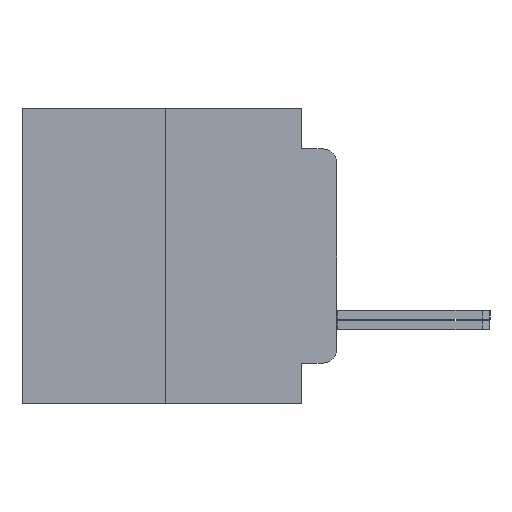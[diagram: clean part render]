
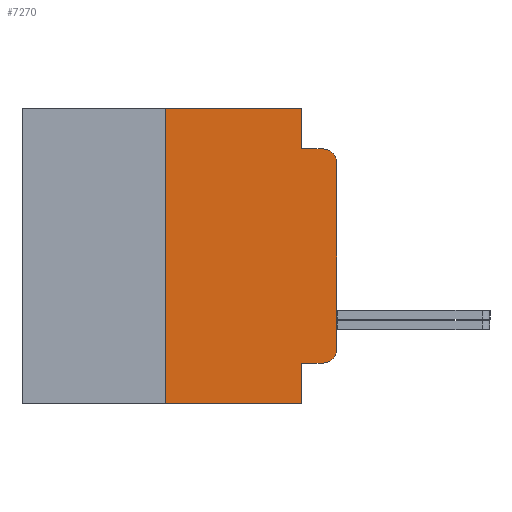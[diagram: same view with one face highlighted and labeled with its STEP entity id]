
A CAD part, left-side view. The second image highlights one B-rep face of the part: STEP entity #7270.
In plain terms, the highlighted planar face has unit normal (-1, 0, 0).
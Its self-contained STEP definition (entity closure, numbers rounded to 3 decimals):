
#16 = ORIENTED_EDGE ( 'NONE', *, *, #16278, .F. ) ;
#500 = VECTOR ( 'NONE', #19968, 1000. ) ;
#1050 = VERTEX_POINT ( 'NONE', #5140 ) ;
#1123 = DIRECTION ( 'NONE',  ( -1., 0., 0. ) ) ;
#1240 = LINE ( 'NONE', #16425, #26227 ) ;
#1304 = CARTESIAN_POINT ( 'NONE',  ( -75.603, 0.508, 3.975 ) ) ;
#1332 = DIRECTION ( 'NONE',  ( 0., 0., -1. ) ) ;
#1714 = VECTOR ( 'NONE', #20306, 1000. ) ;
#1726 = EDGE_LOOP ( 'NONE', ( #14615, #13781, #3419, #8044, #22874, #23533, #16, #23222, #14353, #7827 ) ) ;
#1754 = EDGE_CURVE ( 'NONE', #18497, #1050, #1240, .T. ) ;
#1769 = EDGE_CURVE ( 'NONE', #5410, #3903, #19855, .T. ) ;
#2223 = CARTESIAN_POINT ( 'NONE',  ( -75.603, 0.508, -3.467 ) ) ;
#2358 = AXIS2_PLACEMENT_3D ( 'NONE', #11008, #2539, #19736 ) ;
#2510 = DIRECTION ( 'NONE',  ( 0., 0., 1. ) ) ;
#2539 = DIRECTION ( 'NONE',  ( 1., 0., 0. ) ) ;
#2892 = VERTEX_POINT ( 'NONE', #11447 ) ;
#2897 = EDGE_CURVE ( 'NONE', #2892, #20129, #10812, .T. ) ;
#2918 = CARTESIAN_POINT ( 'NONE',  ( -75.603, 11.684, 5.486 ) ) ;
#3394 = CARTESIAN_POINT ( 'NONE',  ( -75.603, 1.295, 0. ) ) ;
#3419 = ORIENTED_EDGE ( 'NONE', *, *, #26412, .T. ) ;
#3886 = CARTESIAN_POINT ( 'NONE',  ( -75.603, 0., -3.467 ) ) ;
#3903 = VERTEX_POINT ( 'NONE', #8338 ) ;
#4357 = DIRECTION ( 'NONE',  ( 0., 0., -1. ) ) ;
#4677 = PLANE ( 'NONE',  #2358 ) ;
#5100 = VERTEX_POINT ( 'NONE', #1304 ) ;
#5140 = CARTESIAN_POINT ( 'NONE',  ( -75.603, 1.295, 3.975 ) ) ;
#5180 = CARTESIAN_POINT ( 'NONE',  ( -75.603, 6.35, 5.486 ) ) ;
#5410 = VERTEX_POINT ( 'NONE', #14984 ) ;
#5668 = DIRECTION ( 'NONE',  ( 0., -1., 0. ) ) ;
#6194 = VERTEX_POINT ( 'NONE', #5180 ) ;
#6343 = LINE ( 'NONE', #11925, #9980 ) ;
#7270 = ADVANCED_FACE ( 'NONE', ( #21815 ), #4677, .F. ) ;
#7750 = CIRCLE ( 'NONE', #20603, 0.508 ) ;
#7827 = ORIENTED_EDGE ( 'NONE', *, *, #10189, .F. ) ;
#8044 = ORIENTED_EDGE ( 'NONE', *, *, #21125, .T. ) ;
#8338 = CARTESIAN_POINT ( 'NONE',  ( -75.603, 0.508, -3.975 ) ) ;
#8949 = CARTESIAN_POINT ( 'NONE',  ( -75.603, 11.684, -5.486 ) ) ;
#9907 = CARTESIAN_POINT ( 'NONE',  ( -75.603, 1.295, -3.975 ) ) ;
#9980 = VECTOR ( 'NONE', #16386, 1000. ) ;
#10189 = EDGE_CURVE ( 'NONE', #5410, #20129, #14374, .T. ) ;
#10620 = CARTESIAN_POINT ( 'NONE',  ( -75.603, 1.295, 5.486 ) ) ;
#10643 = VECTOR ( 'NONE', #5668, 1000. ) ;
#10812 = LINE ( 'NONE', #8949, #500 ) ;
#11008 = CARTESIAN_POINT ( 'NONE',  ( -75.603, 11.684, 5.486 ) ) ;
#11447 = CARTESIAN_POINT ( 'NONE',  ( -75.603, 6.35, -5.486 ) ) ;
#11925 = CARTESIAN_POINT ( 'NONE',  ( -75.603, 6.35, -5.486 ) ) ;
#12013 = LINE ( 'NONE', #2918, #23655 ) ;
#13091 = CARTESIAN_POINT ( 'NONE',  ( -75.603, 1.295, -5.486 ) ) ;
#13522 = AXIS2_PLACEMENT_3D ( 'NONE', #2223, #17132, #4357 ) ;
#13781 = ORIENTED_EDGE ( 'NONE', *, *, #21374, .T. ) ;
#13873 = LINE ( 'NONE', #15267, #22840 ) ;
#13887 = CARTESIAN_POINT ( 'NONE',  ( -75.603, 0.508, 3.467 ) ) ;
#14353 = ORIENTED_EDGE ( 'NONE', *, *, #2897, .T. ) ;
#14374 = LINE ( 'NONE', #3394, #1714 ) ;
#14615 = ORIENTED_EDGE ( 'NONE', *, *, #1769, .T. ) ;
#14984 = CARTESIAN_POINT ( 'NONE',  ( -75.603, 1.295, -3.975 ) ) ;
#15267 = CARTESIAN_POINT ( 'NONE',  ( -75.603, 0., 5.486 ) ) ;
#16019 = CIRCLE ( 'NONE', #13522, 0.508 ) ;
#16025 = DIRECTION ( 'NONE',  ( 0., 0., -1. ) ) ;
#16278 = EDGE_CURVE ( 'NONE', #6194, #18497, #12013, .T. ) ;
#16319 = LINE ( 'NONE', #20404, #10643 ) ;
#16386 = DIRECTION ( 'NONE',  ( 0., 0., 1. ) ) ;
#16425 = CARTESIAN_POINT ( 'NONE',  ( -75.603, 1.295, 0. ) ) ;
#17132 = DIRECTION ( 'NONE',  ( -1., 0., 0. ) ) ;
#18273 = DIRECTION ( 'NONE',  ( 0., -1., 0. ) ) ;
#18497 = VERTEX_POINT ( 'NONE', #10620 ) ;
#19659 = DIRECTION ( 'NONE',  ( 0., -1., 0. ) ) ;
#19736 = DIRECTION ( 'NONE',  ( 0., 0., -1. ) ) ;
#19855 = LINE ( 'NONE', #9907, #25552 ) ;
#19968 = DIRECTION ( 'NONE',  ( 0., -1., 0. ) ) ;
#20129 = VERTEX_POINT ( 'NONE', #13091 ) ;
#20306 = DIRECTION ( 'NONE',  ( 0., 0., -1. ) ) ;
#20404 = CARTESIAN_POINT ( 'NONE',  ( -75.603, 1.295, 3.975 ) ) ;
#20603 = AXIS2_PLACEMENT_3D ( 'NONE', #13887, #1123, #16025 ) ;
#21125 = EDGE_CURVE ( 'NONE', #24992, #5100, #7750, .T. ) ;
#21374 = EDGE_CURVE ( 'NONE', #3903, #26791, #16019, .T. ) ;
#21815 = FACE_OUTER_BOUND ( 'NONE', #1726, .T. ) ;
#22022 = EDGE_CURVE ( 'NONE', #2892, #6194, #6343, .T. ) ;
#22732 = EDGE_CURVE ( 'NONE', #1050, #5100, #16319, .T. ) ;
#22840 = VECTOR ( 'NONE', #2510, 1000. ) ;
#22874 = ORIENTED_EDGE ( 'NONE', *, *, #22732, .F. ) ;
#23222 = ORIENTED_EDGE ( 'NONE', *, *, #22022, .F. ) ;
#23533 = ORIENTED_EDGE ( 'NONE', *, *, #1754, .F. ) ;
#23655 = VECTOR ( 'NONE', #19659, 1000. ) ;
#24841 = CARTESIAN_POINT ( 'NONE',  ( -75.603, 0., 3.467 ) ) ;
#24992 = VERTEX_POINT ( 'NONE', #24841 ) ;
#25552 = VECTOR ( 'NONE', #18273, 1000. ) ;
#26227 = VECTOR ( 'NONE', #1332, 1000. ) ;
#26412 = EDGE_CURVE ( 'NONE', #26791, #24992, #13873, .T. ) ;
#26791 = VERTEX_POINT ( 'NONE', #3886 ) ;
